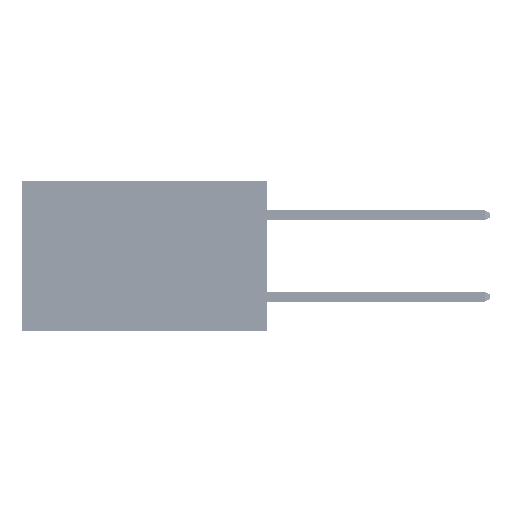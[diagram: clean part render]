
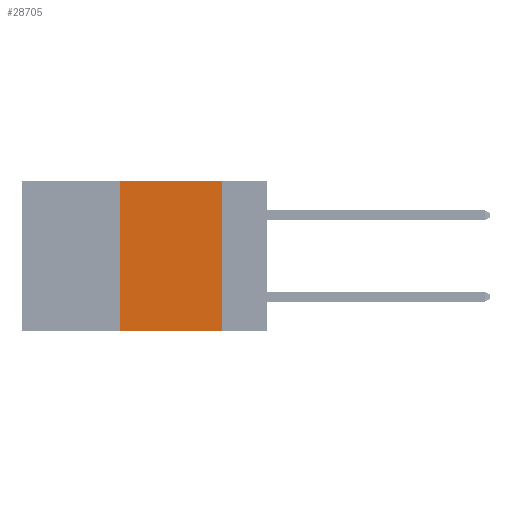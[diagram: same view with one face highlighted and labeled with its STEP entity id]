
A CAD part, left-side view. The second image highlights one B-rep face of the part: STEP entity #28705.
In plain terms, the highlighted planar face has unit normal (-1, 0, 0).
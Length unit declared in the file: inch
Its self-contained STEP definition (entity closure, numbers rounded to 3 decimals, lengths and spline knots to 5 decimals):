
#1086 = CARTESIAN_POINT ( 'NONE',  ( 0., 0.6, 0. ) ) ;
#2470 = ORIENTED_EDGE ( 'NONE', *, *, #43657, .F. ) ;
#2599 = DIRECTION ( 'NONE',  ( 0., -1., 0. ) ) ;
#3368 = EDGE_LOOP ( 'NONE', ( #28917, #2470, #30613, #23863 ) ) ;
#4900 = DIRECTION ( 'NONE',  ( 0., 0., -1. ) ) ;
#5837 = AXIS2_PLACEMENT_3D ( 'NONE', #1086, #46795, #4900 ) ;
#5949 = VECTOR ( 'NONE', #38157, 39.37008 ) ;
#7004 = DIRECTION ( 'NONE',  ( 0., 0., -1. ) ) ;
#9209 = CARTESIAN_POINT ( 'NONE',  ( 0., 0.11, 0. ) ) ;
#11309 = VECTOR ( 'NONE', #13823, 39.37008 ) ;
#13388 = VERTEX_POINT ( 'NONE', #9209 ) ;
#13823 = DIRECTION ( 'NONE',  ( 0., -1., 0. ) ) ;
#15544 = CARTESIAN_POINT ( 'NONE',  ( 0., 0.11, -0.37 ) ) ;
#16399 = VERTEX_POINT ( 'NONE', #15544 ) ;
#18362 = EDGE_CURVE ( 'NONE', #48478, #16399, #24377, .T. ) ;
#19877 = VECTOR ( 'NONE', #2599, 39.37008 ) ;
#21145 = VECTOR ( 'NONE', #7004, 39.37008 ) ;
#21675 = EDGE_CURVE ( 'NONE', #13388, #16399, #33637, .T. ) ;
#21765 = VERTEX_POINT ( 'NONE', #45688 ) ;
#23863 = ORIENTED_EDGE ( 'NONE', *, *, #18362, .T. ) ;
#24377 = LINE ( 'NONE', #28410, #11309 ) ;
#28410 = CARTESIAN_POINT ( 'NONE',  ( 0., 0.6, -0.37 ) ) ;
#28705 = ADVANCED_FACE ( 'NONE', ( #48277 ), #46634, .F. ) ;
#28917 = ORIENTED_EDGE ( 'NONE', *, *, #21675, .F. ) ;
#29589 = CARTESIAN_POINT ( 'NONE',  ( 0., 0.36, -0.37 ) ) ;
#30613 = ORIENTED_EDGE ( 'NONE', *, *, #39060, .F. ) ;
#31472 = LINE ( 'NONE', #41665, #5949 ) ;
#33637 = LINE ( 'NONE', #37716, #21145 ) ;
#37716 = CARTESIAN_POINT ( 'NONE',  ( 0., 0.11, 0. ) ) ;
#38157 = DIRECTION ( 'NONE',  ( 0., 0., 1. ) ) ;
#39060 = EDGE_CURVE ( 'NONE', #48478, #21765, #31472, .T. ) ;
#40486 = CARTESIAN_POINT ( 'NONE',  ( 0., 0.6, 0. ) ) ;
#41665 = CARTESIAN_POINT ( 'NONE',  ( 0., 0.36, 0. ) ) ;
#43037 = LINE ( 'NONE', #40486, #19877 ) ;
#43657 = EDGE_CURVE ( 'NONE', #21765, #13388, #43037, .T. ) ;
#45688 = CARTESIAN_POINT ( 'NONE',  ( 0., 0.36, 0. ) ) ;
#46634 = PLANE ( 'NONE',  #5837 ) ;
#46795 = DIRECTION ( 'NONE',  ( 1., 0., 0. ) ) ;
#48277 = FACE_OUTER_BOUND ( 'NONE', #3368, .T. ) ;
#48478 = VERTEX_POINT ( 'NONE', #29589 ) ;
